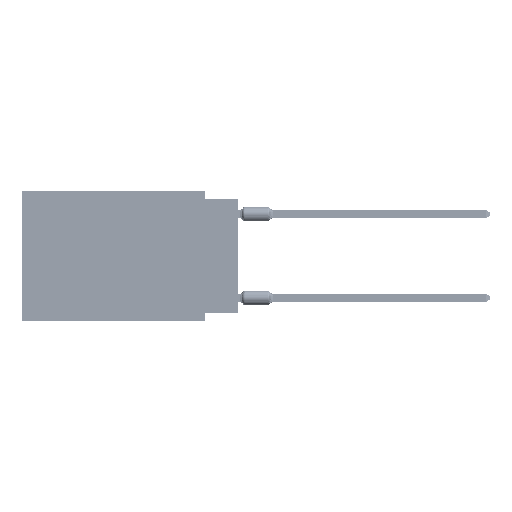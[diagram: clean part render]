
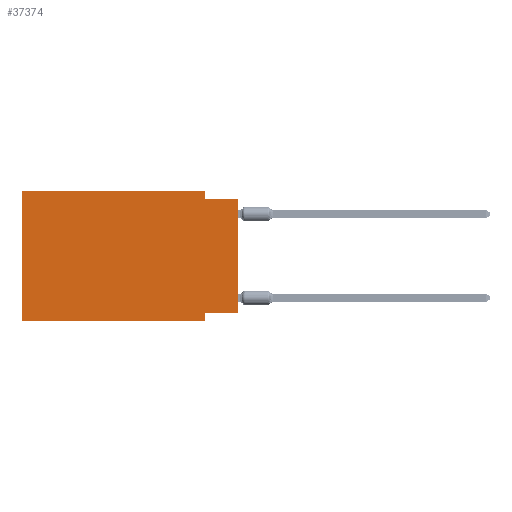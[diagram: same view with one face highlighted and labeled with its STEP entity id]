
A CAD part, left-side view. The second image highlights one B-rep face of the part: STEP entity #37374.
In plain terms, the highlighted planar face has unit normal (-1, 0, 0).
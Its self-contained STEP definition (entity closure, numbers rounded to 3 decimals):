
#770 = CARTESIAN_POINT ( 'NONE',  ( 0., 2.54, 0. ) ) ;
#1676 = CARTESIAN_POINT ( 'NONE',  ( 0., 16.383, 0. ) ) ;
#2338 = VECTOR ( 'NONE', #36503, 1000. ) ;
#2397 = CARTESIAN_POINT ( 'NONE',  ( 0., 2.54, -9.906 ) ) ;
#3594 = DIRECTION ( 'NONE',  ( 0., 0., 1. ) ) ;
#4424 = LINE ( 'NONE', #29230, #59334 ) ;
#4681 = VECTOR ( 'NONE', #20159, 1000. ) ;
#6243 = EDGE_CURVE ( 'NONE', #10709, #27302, #71393, .T. ) ;
#6301 = CARTESIAN_POINT ( 'NONE',  ( 0., 0., -0.635 ) ) ;
#6316 = CARTESIAN_POINT ( 'NONE',  ( 0., 16.383, 0. ) ) ;
#10672 = CARTESIAN_POINT ( 'NONE',  ( 0., 2.54, -0.635 ) ) ;
#10709 = VERTEX_POINT ( 'NONE', #73598 ) ;
#11275 = LINE ( 'NONE', #6301, #2338 ) ;
#11561 = ORIENTED_EDGE ( 'NONE', *, *, #37799, .T. ) ;
#11991 = LINE ( 'NONE', #42596, #26246 ) ;
#12093 = DIRECTION ( 'NONE',  ( 0., 0., -1. ) ) ;
#12744 = LINE ( 'NONE', #770, #4681 ) ;
#18441 = EDGE_CURVE ( 'NONE', #44228, #58329, #12744, .T. ) ;
#19195 = VERTEX_POINT ( 'NONE', #61347 ) ;
#20159 = DIRECTION ( 'NONE',  ( 0., 0., -1. ) ) ;
#24235 = VECTOR ( 'NONE', #62998, 1000. ) ;
#25737 = FACE_OUTER_BOUND ( 'NONE', #27284, .T. ) ;
#26246 = VECTOR ( 'NONE', #69418, 1000. ) ;
#26479 = DIRECTION ( 'NONE',  ( 0., 0., 1. ) ) ;
#27284 = EDGE_LOOP ( 'NONE', ( #58846, #74128, #30557, #57823, #28550, #11561, #67657, #40929 ) ) ;
#27302 = VERTEX_POINT ( 'NONE', #75443 ) ;
#28550 = ORIENTED_EDGE ( 'NONE', *, *, #79954, .F. ) ;
#29230 = CARTESIAN_POINT ( 'NONE',  ( 0., 0., 0. ) ) ;
#29843 = VERTEX_POINT ( 'NONE', #55530 ) ;
#29981 = CARTESIAN_POINT ( 'NONE',  ( 0., 0., -0.635 ) ) ;
#30557 = ORIENTED_EDGE ( 'NONE', *, *, #18441, .F. ) ;
#34315 = LINE ( 'NONE', #1676, #77503 ) ;
#36207 = EDGE_CURVE ( 'NONE', #58329, #76860, #11275, .T. ) ;
#36503 = DIRECTION ( 'NONE',  ( 0., -1., 0. ) ) ;
#36920 = DIRECTION ( 'NONE',  ( 1., 0., 0. ) ) ;
#37374 = ADVANCED_FACE ( 'NONE', ( #25737 ), #63350, .F. ) ;
#37799 = EDGE_CURVE ( 'NONE', #19195, #27302, #11991, .T. ) ;
#38206 = LINE ( 'NONE', #43972, #24235 ) ;
#40929 = ORIENTED_EDGE ( 'NONE', *, *, #53941, .F. ) ;
#42193 = CARTESIAN_POINT ( 'NONE',  ( 0., 2.54, 0. ) ) ;
#42596 = CARTESIAN_POINT ( 'NONE',  ( 0., 16.383, -9.906 ) ) ;
#43972 = CARTESIAN_POINT ( 'NONE',  ( 0., 0., -9.271 ) ) ;
#44228 = VERTEX_POINT ( 'NONE', #42193 ) ;
#51871 = VECTOR ( 'NONE', #80055, 1000. ) ;
#53941 = EDGE_CURVE ( 'NONE', #55592, #10709, #38206, .T. ) ;
#55530 = CARTESIAN_POINT ( 'NONE',  ( 0., 16.383, 0. ) ) ;
#55592 = VERTEX_POINT ( 'NONE', #75663 ) ;
#57823 = ORIENTED_EDGE ( 'NONE', *, *, #66607, .F. ) ;
#58329 = VERTEX_POINT ( 'NONE', #10672 ) ;
#58846 = ORIENTED_EDGE ( 'NONE', *, *, #62717, .T. ) ;
#59213 = AXIS2_PLACEMENT_3D ( 'NONE', #6316, #36920, #12093 ) ;
#59334 = VECTOR ( 'NONE', #3594, 1000. ) ;
#61090 = CARTESIAN_POINT ( 'NONE',  ( 0., 16.383, 0. ) ) ;
#61347 = CARTESIAN_POINT ( 'NONE',  ( 0., 16.383, -9.906 ) ) ;
#62717 = EDGE_CURVE ( 'NONE', #55592, #76860, #4424, .T. ) ;
#62998 = DIRECTION ( 'NONE',  ( 0., 1., 0. ) ) ;
#63350 = PLANE ( 'NONE',  #59213 ) ;
#66607 = EDGE_CURVE ( 'NONE', #29843, #44228, #68082, .T. ) ;
#67657 = ORIENTED_EDGE ( 'NONE', *, *, #6243, .F. ) ;
#68082 = LINE ( 'NONE', #61090, #51871 ) ;
#69418 = DIRECTION ( 'NONE',  ( 0., -1., 0. ) ) ;
#69825 = VECTOR ( 'NONE', #72598, 1000. ) ;
#71393 = LINE ( 'NONE', #2397, #69825 ) ;
#72598 = DIRECTION ( 'NONE',  ( 0., 0., -1. ) ) ;
#73598 = CARTESIAN_POINT ( 'NONE',  ( 0., 2.54, -9.271 ) ) ;
#74128 = ORIENTED_EDGE ( 'NONE', *, *, #36207, .F. ) ;
#75443 = CARTESIAN_POINT ( 'NONE',  ( 0., 2.54, -9.906 ) ) ;
#75663 = CARTESIAN_POINT ( 'NONE',  ( 0., 0., -9.271 ) ) ;
#76860 = VERTEX_POINT ( 'NONE', #29981 ) ;
#77503 = VECTOR ( 'NONE', #26479, 1000. ) ;
#79954 = EDGE_CURVE ( 'NONE', #19195, #29843, #34315, .T. ) ;
#80055 = DIRECTION ( 'NONE',  ( 0., -1., 0. ) ) ;
